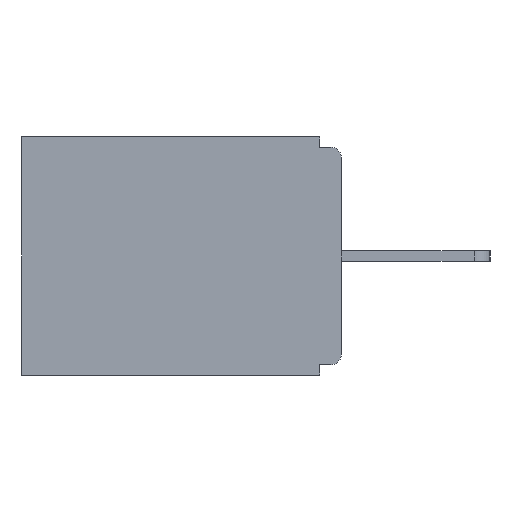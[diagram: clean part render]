
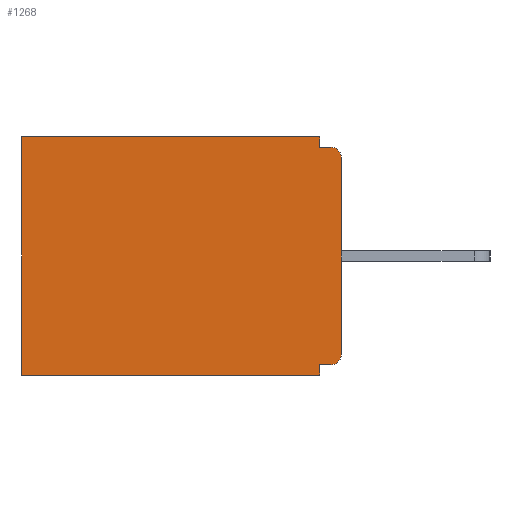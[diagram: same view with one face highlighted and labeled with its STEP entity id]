
A CAD part, left-side view. The second image highlights one B-rep face of the part: STEP entity #1268.
In plain terms, the highlighted planar face has unit normal (-1, 0, 0).
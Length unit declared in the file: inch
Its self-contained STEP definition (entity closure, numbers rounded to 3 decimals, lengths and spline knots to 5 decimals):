
#460 = EDGE_CURVE ( 'NONE', #2867, #16244, #9731, .T. ) ;
#564 = DIRECTION ( 'NONE',  ( 0., -1., 0. ) ) ;
#587 = VERTEX_POINT ( 'NONE', #20409 ) ;
#1098 = CARTESIAN_POINT ( 'NONE',  ( 0.298, 0., 0. ) ) ;
#1119 = CARTESIAN_POINT ( 'NONE',  ( 0.298, 0.015, -0.328 ) ) ;
#1268 = ADVANCED_FACE ( 'NONE', ( #4340 ), #10810, .F. ) ;
#1402 = CARTESIAN_POINT ( 'NONE',  ( 0.298, 0.015, -0.313 ) ) ;
#1481 = CARTESIAN_POINT ( 'NONE',  ( 0.298, 0.015, -0.03 ) ) ;
#2165 = ORIENTED_EDGE ( 'NONE', *, *, #460, .F. ) ;
#2281 = CARTESIAN_POINT ( 'NONE',  ( 0.298, 0., 0. ) ) ;
#2353 = CARTESIAN_POINT ( 'NONE',  ( 0.298, 0., 0. ) ) ;
#2867 = VERTEX_POINT ( 'NONE', #14941 ) ;
#3042 = EDGE_CURVE ( 'NONE', #21811, #5295, #12008, .T. ) ;
#3156 = CARTESIAN_POINT ( 'NONE',  ( 0.298, 0.46, 0. ) ) ;
#3256 = ORIENTED_EDGE ( 'NONE', *, *, #15219, .T. ) ;
#3581 = ORIENTED_EDGE ( 'NONE', *, *, #10326, .T. ) ;
#3684 = VERTEX_POINT ( 'NONE', #12891 ) ;
#4340 = FACE_OUTER_BOUND ( 'NONE', #7219, .T. ) ;
#4850 = VECTOR ( 'NONE', #564, 39.37008 ) ;
#4942 = DIRECTION ( 'NONE',  ( 0., 0., -1. ) ) ;
#5127 = DIRECTION ( 'NONE',  ( -1., 0., 0. ) ) ;
#5233 = CARTESIAN_POINT ( 'NONE',  ( 0.298, 0.031, -0.343 ) ) ;
#5264 = DIRECTION ( 'NONE',  ( 0., 1., 0. ) ) ;
#5295 = VERTEX_POINT ( 'NONE', #7080 ) ;
#5447 = AXIS2_PLACEMENT_3D ( 'NONE', #2353, #12594, #9136 ) ;
#5602 = EDGE_CURVE ( 'NONE', #11120, #17574, #20147, .T. ) ;
#5607 = ORIENTED_EDGE ( 'NONE', *, *, #18424, .F. ) ;
#5852 = VECTOR ( 'NONE', #7389, 39.37008 ) ;
#5922 = AXIS2_PLACEMENT_3D ( 'NONE', #1481, #5127, #8589 ) ;
#6131 = VECTOR ( 'NONE', #6181, 39.37008 ) ;
#6181 = DIRECTION ( 'NONE',  ( 0., 0., -1. ) ) ;
#6199 = CARTESIAN_POINT ( 'NONE',  ( 0.298, 0.46, 0. ) ) ;
#6444 = VECTOR ( 'NONE', #7699, 39.37008 ) ;
#6868 = ORIENTED_EDGE ( 'NONE', *, *, #12701, .F. ) ;
#6914 = VERTEX_POINT ( 'NONE', #6199 ) ;
#7080 = CARTESIAN_POINT ( 'NONE',  ( 0.298, 0.015, -0.015 ) ) ;
#7199 = VECTOR ( 'NONE', #19985, 39.37008 ) ;
#7219 = EDGE_LOOP ( 'NONE', ( #17212, #5607, #2165, #3256, #3581, #16262, #14610, #14473, #14126, #6868 ) ) ;
#7389 = DIRECTION ( 'NONE',  ( 0., 1., 0. ) ) ;
#7699 = DIRECTION ( 'NONE',  ( 0., 0., -1. ) ) ;
#8202 = CARTESIAN_POINT ( 'NONE',  ( 0.298, 0., -0.343 ) ) ;
#8505 = LINE ( 'NONE', #15291, #18225 ) ;
#8589 = DIRECTION ( 'NONE',  ( 0., 0., -1. ) ) ;
#9136 = DIRECTION ( 'NONE',  ( 0., 0., -1. ) ) ;
#9539 = LINE ( 'NONE', #1098, #6131 ) ;
#9731 = LINE ( 'NONE', #13635, #10698 ) ;
#10326 = EDGE_CURVE ( 'NONE', #6914, #587, #20284, .T. ) ;
#10687 = EDGE_CURVE ( 'NONE', #3684, #10772, #14494, .T. ) ;
#10698 = VECTOR ( 'NONE', #11637, 39.37008 ) ;
#10772 = VERTEX_POINT ( 'NONE', #5233 ) ;
#10810 = PLANE ( 'NONE',  #5447 ) ;
#11046 = CARTESIAN_POINT ( 'NONE',  ( 0.298, 0.031, -0.343 ) ) ;
#11120 = VERTEX_POINT ( 'NONE', #1119 ) ;
#11594 = EDGE_CURVE ( 'NONE', #11120, #3684, #8505, .T. ) ;
#11637 = DIRECTION ( 'NONE',  ( 0., 0., -1. ) ) ;
#11730 = DIRECTION ( 'NONE',  ( 0., 0., -1. ) ) ;
#12008 = CIRCLE ( 'NONE', #5922, 0.015 ) ;
#12594 = DIRECTION ( 'NONE',  ( 1., 0., 0. ) ) ;
#12701 = EDGE_CURVE ( 'NONE', #21811, #17574, #9539, .T. ) ;
#12732 = EDGE_CURVE ( 'NONE', #10772, #587, #15321, .T. ) ;
#12891 = CARTESIAN_POINT ( 'NONE',  ( 0.298, 0.031, -0.328 ) ) ;
#13635 = CARTESIAN_POINT ( 'NONE',  ( 0.298, 0.031, -0.343 ) ) ;
#13979 = CARTESIAN_POINT ( 'NONE',  ( 0.298, 0.031, -0.015 ) ) ;
#14126 = ORIENTED_EDGE ( 'NONE', *, *, #5602, .T. ) ;
#14473 = ORIENTED_EDGE ( 'NONE', *, *, #11594, .F. ) ;
#14494 = LINE ( 'NONE', #11046, #6444 ) ;
#14610 = ORIENTED_EDGE ( 'NONE', *, *, #10687, .F. ) ;
#14941 = CARTESIAN_POINT ( 'NONE',  ( 0.298, 0.031, 0. ) ) ;
#15219 = EDGE_CURVE ( 'NONE', #2867, #6914, #17507, .T. ) ;
#15291 = CARTESIAN_POINT ( 'NONE',  ( 0.298, 0., -0.328 ) ) ;
#15321 = LINE ( 'NONE', #8202, #7199 ) ;
#16128 = LINE ( 'NONE', #16233, #4850 ) ;
#16233 = CARTESIAN_POINT ( 'NONE',  ( 0.298, 0., -0.015 ) ) ;
#16244 = VERTEX_POINT ( 'NONE', #13979 ) ;
#16262 = ORIENTED_EDGE ( 'NONE', *, *, #12732, .F. ) ;
#17212 = ORIENTED_EDGE ( 'NONE', *, *, #3042, .T. ) ;
#17507 = LINE ( 'NONE', #2281, #5852 ) ;
#17574 = VERTEX_POINT ( 'NONE', #19532 ) ;
#18191 = VECTOR ( 'NONE', #11730, 39.37008 ) ;
#18225 = VECTOR ( 'NONE', #5264, 39.37008 ) ;
#18424 = EDGE_CURVE ( 'NONE', #16244, #5295, #16128, .T. ) ;
#19532 = CARTESIAN_POINT ( 'NONE',  ( 0.298, 0., -0.313 ) ) ;
#19985 = DIRECTION ( 'NONE',  ( 0., 1., 0. ) ) ;
#20147 = CIRCLE ( 'NONE', #21934, 0.015 ) ;
#20284 = LINE ( 'NONE', #3156, #18191 ) ;
#20409 = CARTESIAN_POINT ( 'NONE',  ( 0.298, 0.46, -0.343 ) ) ;
#20461 = CARTESIAN_POINT ( 'NONE',  ( 0.298, 0., -0.03 ) ) ;
#21811 = VERTEX_POINT ( 'NONE', #20461 ) ;
#21862 = DIRECTION ( 'NONE',  ( -1., 0., 0. ) ) ;
#21934 = AXIS2_PLACEMENT_3D ( 'NONE', #1402, #21862, #4942 ) ;
